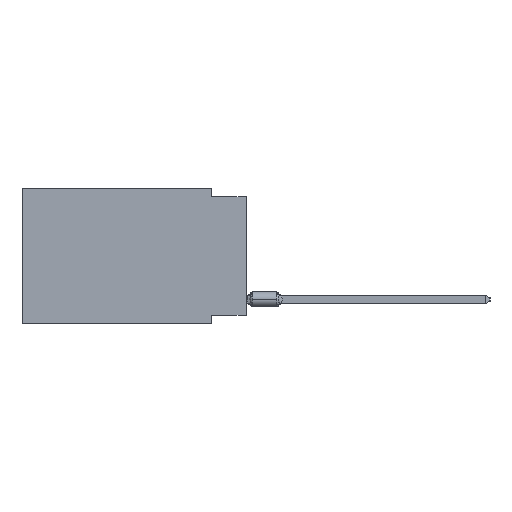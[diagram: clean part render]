
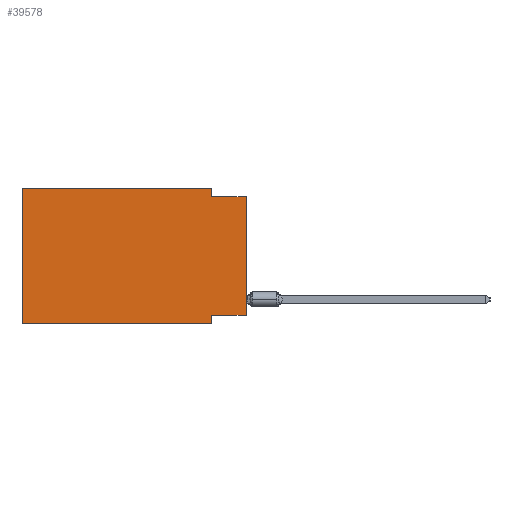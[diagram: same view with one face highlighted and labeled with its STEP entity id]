
A CAD part, left-side view. The second image highlights one B-rep face of the part: STEP entity #39578.
In plain terms, the highlighted planar face has unit normal (-1, 0, 0).
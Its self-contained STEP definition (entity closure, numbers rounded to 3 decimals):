
#808 = EDGE_CURVE ( 'NONE', #37899, #57822, #8123, .T. ) ;
#2022 = DIRECTION ( 'NONE',  ( 0., 0., 1. ) ) ;
#4638 = CARTESIAN_POINT ( 'NONE',  ( 0., 2.54, 0. ) ) ;
#4901 = EDGE_CURVE ( 'NONE', #19699, #38201, #21646, .T. ) ;
#5722 = CARTESIAN_POINT ( 'NONE',  ( 0., 2.54, 0. ) ) ;
#6431 = ORIENTED_EDGE ( 'NONE', *, *, #808, .F. ) ;
#8123 = LINE ( 'NONE', #26420, #27911 ) ;
#8405 = LINE ( 'NONE', #13229, #25921 ) ;
#8415 = LINE ( 'NONE', #18997, #9357 ) ;
#9357 = VECTOR ( 'NONE', #62939, 1000. ) ;
#9878 = DIRECTION ( 'NONE',  ( 0., 1., 0. ) ) ;
#11711 = CARTESIAN_POINT ( 'NONE',  ( 0., 2.54, -0.635 ) ) ;
#12633 = DIRECTION ( 'NONE',  ( 0., 0., 1. ) ) ;
#13229 = CARTESIAN_POINT ( 'NONE',  ( 0., 16.383, -9.906 ) ) ;
#13344 = CARTESIAN_POINT ( 'NONE',  ( 0., 2.54, -9.906 ) ) ;
#14778 = VECTOR ( 'NONE', #49868, 1000. ) ;
#16517 = CARTESIAN_POINT ( 'NONE',  ( 0., 0., 0. ) ) ;
#16613 = VECTOR ( 'NONE', #12633, 1000. ) ;
#18154 = ORIENTED_EDGE ( 'NONE', *, *, #57890, .T. ) ;
#18607 = EDGE_CURVE ( 'NONE', #21623, #23788, #30612, .T. ) ;
#18997 = CARTESIAN_POINT ( 'NONE',  ( 0., 0., -0.635 ) ) ;
#19699 = VERTEX_POINT ( 'NONE', #46381 ) ;
#20228 = ORIENTED_EDGE ( 'NONE', *, *, #18607, .F. ) ;
#20767 = LINE ( 'NONE', #49642, #29260 ) ;
#21016 = EDGE_CURVE ( 'NONE', #23788, #38201, #8415, .T. ) ;
#21157 = AXIS2_PLACEMENT_3D ( 'NONE', #56035, #26841, #50584 ) ;
#21380 = VERTEX_POINT ( 'NONE', #51642 ) ;
#21623 = VERTEX_POINT ( 'NONE', #5722 ) ;
#21646 = LINE ( 'NONE', #16517, #16613 ) ;
#22889 = DIRECTION ( 'NONE',  ( 0., -1., 0. ) ) ;
#23223 = LINE ( 'NONE', #43128, #23352 ) ;
#23352 = VECTOR ( 'NONE', #22889, 1000. ) ;
#23575 = ORIENTED_EDGE ( 'NONE', *, *, #4901, .T. ) ;
#23606 = LINE ( 'NONE', #13344, #58884 ) ;
#23788 = VERTEX_POINT ( 'NONE', #11711 ) ;
#25921 = VECTOR ( 'NONE', #57498, 1000. ) ;
#26420 = CARTESIAN_POINT ( 'NONE',  ( 0., 16.383, 0. ) ) ;
#26841 = DIRECTION ( 'NONE',  ( 1., 0., 0. ) ) ;
#27911 = VECTOR ( 'NONE', #2022, 1000. ) ;
#29260 = VECTOR ( 'NONE', #9878, 1000. ) ;
#30612 = LINE ( 'NONE', #4638, #14778 ) ;
#33191 = DIRECTION ( 'NONE',  ( 0., 0., -1. ) ) ;
#36174 = EDGE_CURVE ( 'NONE', #57822, #21623, #23223, .T. ) ;
#37821 = ORIENTED_EDGE ( 'NONE', *, *, #48699, .F. ) ;
#37899 = VERTEX_POINT ( 'NONE', #63464 ) ;
#38201 = VERTEX_POINT ( 'NONE', #61849 ) ;
#39578 = ADVANCED_FACE ( 'NONE', ( #45170 ), #55417, .F. ) ;
#40874 = EDGE_CURVE ( 'NONE', #19699, #21380, #20767, .T. ) ;
#41959 = CARTESIAN_POINT ( 'NONE',  ( 0., 2.54, -9.906 ) ) ;
#42951 = ORIENTED_EDGE ( 'NONE', *, *, #36174, .F. ) ;
#43128 = CARTESIAN_POINT ( 'NONE',  ( 0., 16.383, 0. ) ) ;
#44092 = ORIENTED_EDGE ( 'NONE', *, *, #21016, .F. ) ;
#44655 = ORIENTED_EDGE ( 'NONE', *, *, #40874, .F. ) ;
#45170 = FACE_OUTER_BOUND ( 'NONE', #50742, .T. ) ;
#46381 = CARTESIAN_POINT ( 'NONE',  ( 0., 0., -9.271 ) ) ;
#48699 = EDGE_CURVE ( 'NONE', #21380, #58599, #23606, .T. ) ;
#49642 = CARTESIAN_POINT ( 'NONE',  ( 0., 0., -9.271 ) ) ;
#49868 = DIRECTION ( 'NONE',  ( 0., 0., -1. ) ) ;
#50584 = DIRECTION ( 'NONE',  ( 0., 0., -1. ) ) ;
#50742 = EDGE_LOOP ( 'NONE', ( #23575, #44092, #20228, #42951, #6431, #18154, #37821, #44655 ) ) ;
#51642 = CARTESIAN_POINT ( 'NONE',  ( 0., 2.54, -9.271 ) ) ;
#52039 = CARTESIAN_POINT ( 'NONE',  ( 0., 16.383, 0. ) ) ;
#55417 = PLANE ( 'NONE',  #21157 ) ;
#56035 = CARTESIAN_POINT ( 'NONE',  ( 0., 16.383, 0. ) ) ;
#57498 = DIRECTION ( 'NONE',  ( 0., -1., 0. ) ) ;
#57822 = VERTEX_POINT ( 'NONE', #52039 ) ;
#57890 = EDGE_CURVE ( 'NONE', #37899, #58599, #8405, .T. ) ;
#58599 = VERTEX_POINT ( 'NONE', #41959 ) ;
#58884 = VECTOR ( 'NONE', #33191, 1000. ) ;
#61849 = CARTESIAN_POINT ( 'NONE',  ( 0., 0., -0.635 ) ) ;
#62939 = DIRECTION ( 'NONE',  ( 0., -1., 0. ) ) ;
#63464 = CARTESIAN_POINT ( 'NONE',  ( 0., 16.383, -9.906 ) ) ;
